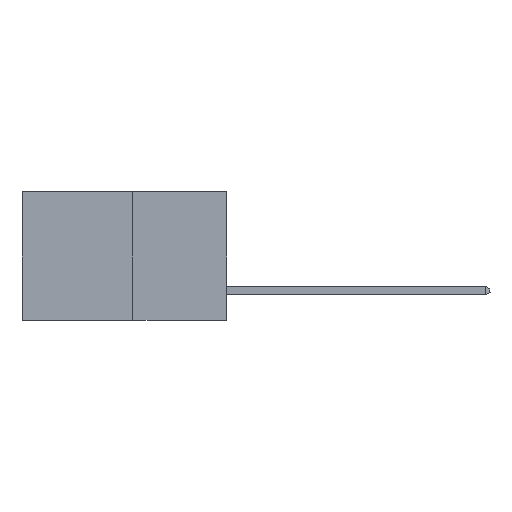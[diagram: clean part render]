
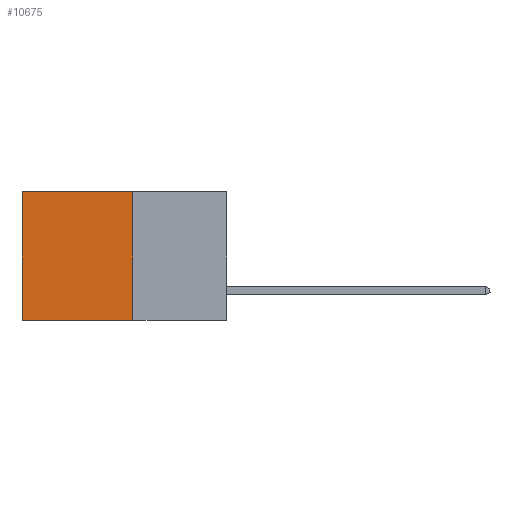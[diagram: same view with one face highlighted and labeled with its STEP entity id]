
A CAD part, left-side view. The second image highlights one B-rep face of the part: STEP entity #10675.
In plain terms, the highlighted planar face has unit normal (-1, 0, 0).
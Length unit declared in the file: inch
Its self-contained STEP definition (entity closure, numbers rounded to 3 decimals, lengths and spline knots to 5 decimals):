
#209 = FACE_OUTER_BOUND ( 'NONE', #4743, .T. ) ;
#731 = CARTESIAN_POINT ( 'NONE',  ( 0.277, 0.59, 0. ) ) ;
#819 = VECTOR ( 'NONE', #2175, 39.37008 ) ;
#910 = VECTOR ( 'NONE', #10885, 39.37008 ) ;
#1186 = ORIENTED_EDGE ( 'NONE', *, *, #11249, .T. ) ;
#1282 = DIRECTION ( 'NONE',  ( 1., 0., 0. ) ) ;
#1418 = CARTESIAN_POINT ( 'NONE',  ( 0.277, 0.27, 0. ) ) ;
#1686 = ORIENTED_EDGE ( 'NONE', *, *, #2377, .T. ) ;
#2032 = ORIENTED_EDGE ( 'NONE', *, *, #12243, .F. ) ;
#2121 = CARTESIAN_POINT ( 'NONE',  ( 0.277, 0.59, -0.37 ) ) ;
#2175 = DIRECTION ( 'NONE',  ( 0., 0., -1. ) ) ;
#2294 = CARTESIAN_POINT ( 'NONE',  ( 0.277, 0.59, -0.37 ) ) ;
#2377 = EDGE_CURVE ( 'NONE', #6978, #4939, #3751, .T. ) ;
#3159 = VERTEX_POINT ( 'NONE', #10126 ) ;
#3751 = LINE ( 'NONE', #2294, #819 ) ;
#4646 = LINE ( 'NONE', #11599, #10072 ) ;
#4743 = EDGE_LOOP ( 'NONE', ( #1686, #2032, #11645, #1186 ) ) ;
#4939 = VERTEX_POINT ( 'NONE', #2121 ) ;
#5654 = CARTESIAN_POINT ( 'NONE',  ( 0.277, 0.27, -0.37 ) ) ;
#6321 = DIRECTION ( 'NONE',  ( 0., 1., 0. ) ) ;
#6609 = CARTESIAN_POINT ( 'NONE',  ( 0.277, 0.27, 0. ) ) ;
#6774 = LINE ( 'NONE', #6609, #910 ) ;
#6978 = VERTEX_POINT ( 'NONE', #731 ) ;
#7450 = LINE ( 'NONE', #9990, #10266 ) ;
#7851 = PLANE ( 'NONE',  #13121 ) ;
#8917 = DIRECTION ( 'NONE',  ( 0., 0., -1. ) ) ;
#9537 = VERTEX_POINT ( 'NONE', #1418 ) ;
#9990 = CARTESIAN_POINT ( 'NONE',  ( 0.277, 0.27, -0.37 ) ) ;
#10072 = VECTOR ( 'NONE', #6321, 39.37008 ) ;
#10126 = CARTESIAN_POINT ( 'NONE',  ( 0.277, 0.27, -0.37 ) ) ;
#10157 = EDGE_CURVE ( 'NONE', #9537, #3159, #7450, .T. ) ;
#10266 = VECTOR ( 'NONE', #11056, 39.37008 ) ;
#10675 = ADVANCED_FACE ( 'NONE', ( #209 ), #7851, .F. ) ;
#10885 = DIRECTION ( 'NONE',  ( 0., 1., 0. ) ) ;
#11056 = DIRECTION ( 'NONE',  ( 0., 0., -1. ) ) ;
#11249 = EDGE_CURVE ( 'NONE', #9537, #6978, #6774, .T. ) ;
#11599 = CARTESIAN_POINT ( 'NONE',  ( 0.277, 0.27, -0.37 ) ) ;
#11645 = ORIENTED_EDGE ( 'NONE', *, *, #10157, .F. ) ;
#12243 = EDGE_CURVE ( 'NONE', #3159, #4939, #4646, .T. ) ;
#13121 = AXIS2_PLACEMENT_3D ( 'NONE', #5654, #1282, #8917 ) ;
